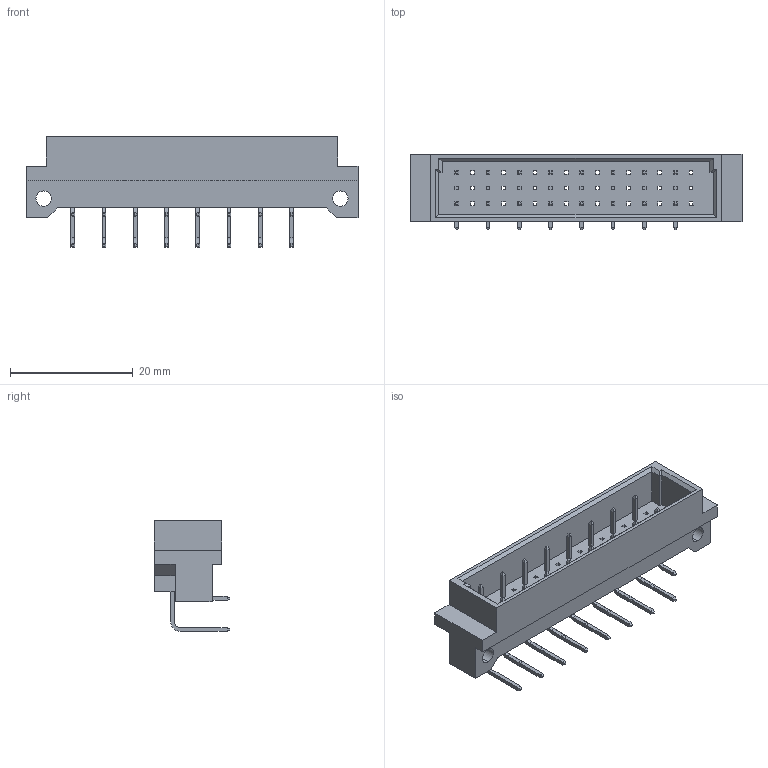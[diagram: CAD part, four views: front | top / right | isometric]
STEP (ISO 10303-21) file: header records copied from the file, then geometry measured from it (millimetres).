
FILE_DESCRIPTION (( 'STEP AP214' ), '1' );
FILE_NAME ('495-016-660-622.STEP', '2020-08-12T14:15:32', ( '' ), ( '' ), 'SwSTEP 2.0', 'SolidWorks 2020', '' );
FILE_SCHEMA (( 'AUTOMOTIVE_DESIGN' ));
Length unit declared in the file: millimetre
Products named in the file (4): 495 Part_48; 495-290-3; 495-290-1; 495-016-660-622
Assembly tree (17 placements, depth 2):
  495-016-660-622
    495 Part_48
    495-290-1  x8
    495-290-3  x8
Bounding box: 54 x 12.27 x 18.05 mm (x, y, z)
Volume: 3564.8 mm3; surface area: 4729.5 mm2
Topology: 17 solids, 17 shells, 530 faces, 1344 edges, 850 vertices
Faces by surface type: plane 494, cylinder 36
Entity records: 9242 total; most frequent: CARTESIAN_POINT 1596, ORIENTED_EDGE 1568, DIRECTION 1396, EDGE_CURVE 784, VECTOR 768, LINE 768, VERTEX_POINT 514, EDGE_LOOP 380
